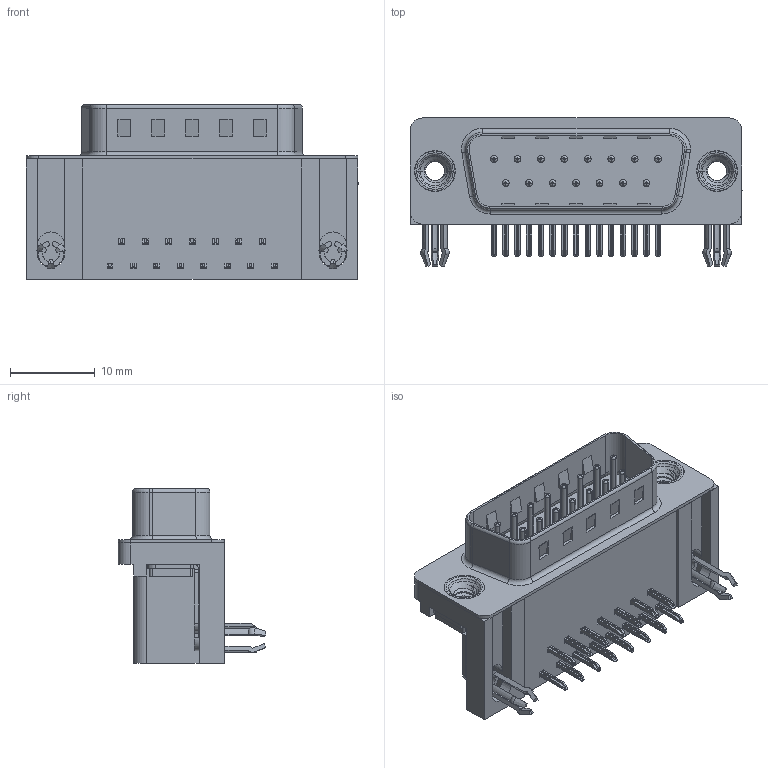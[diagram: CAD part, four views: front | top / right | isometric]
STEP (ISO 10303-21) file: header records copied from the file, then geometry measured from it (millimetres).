
FILE_DESCRIPTION (( 'STEP AP203' ), '1' );
FILE_NAME ('629-015-240-042.STEP', '2021-09-21T20:07:12', ( '' ), ( '' ), 'SwSTEP 2.0', 'SolidWorks 2020', '' );
FILE_SCHEMA (( 'CONFIG_CONTROL_DESIGN' ));
Length unit declared in the file: millimetre
Products named in the file (7): 629 Shell_15 Socket; 629 4-40 Threaded Rivet; 629 Contact Bottom; 629-015-240-042; 629 Housing_15 Socket; 629 3 Prong Board Lock; 629 Contact Top
Assembly tree (21 placements, depth 2):
  629-015-240-042
    629 Housing_15 Socket
    629 Shell_15 Socket
    629 Contact Bottom  x7
    629 Contact Top  x8
    629 3 Prong Board Lock  x2
    629 4-40 Threaded Rivet  x2
Bounding box: 39.22 x 17.48 x 20.6 mm (x, y, z)
Volume: 5090.4 mm3; surface area: 6133.4 mm2
Topology: 21 solids, 21 shells, 1579 faces, 3981 edges, 2481 vertices
Faces by surface type: plane 929, cylinder 451, torus 145, cone 48, bspline 6
Entity records: 20688 total; most frequent: CARTESIAN_POINT 4881, DIRECTION 3140, ORIENTED_EDGE 3006, EDGE_CURVE 1503, AXIS2_PLACEMENT_3D 1072, VECTOR 996, LINE 996, VERTEX_POINT 963
